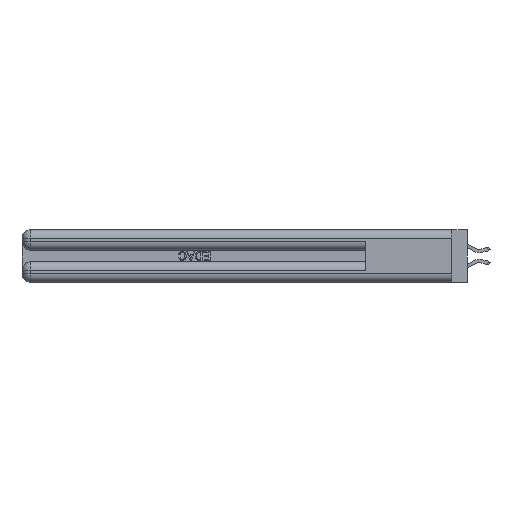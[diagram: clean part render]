
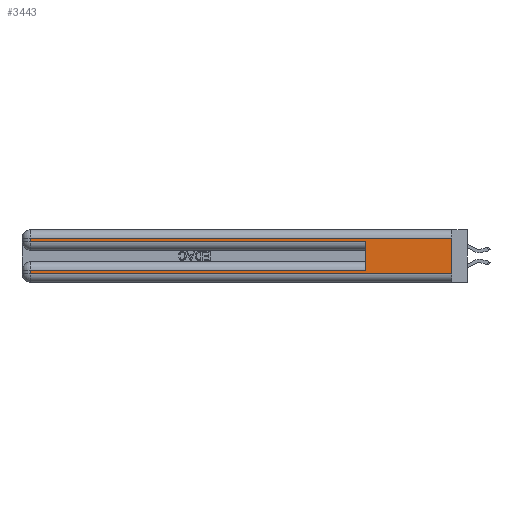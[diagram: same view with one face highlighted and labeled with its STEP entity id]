
A CAD part, left-side view. The second image highlights one B-rep face of the part: STEP entity #3443.
In plain terms, the highlighted planar face has unit normal (-1, 0, 0).
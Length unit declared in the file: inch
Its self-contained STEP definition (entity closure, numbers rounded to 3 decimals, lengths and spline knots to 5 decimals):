
#501 = EDGE_CURVE ( 'NONE', #843, #32070, #34687, .T. ) ;
#601 = CARTESIAN_POINT ( 'NONE',  ( 0., 2.94, 0.37 ) ) ;
#843 = VERTEX_POINT ( 'NONE', #7015 ) ;
#874 = DIRECTION ( 'NONE',  ( 1., 0., 0. ) ) ;
#916 = VECTOR ( 'NONE', #10515, 39.37008 ) ;
#2518 = LINE ( 'NONE', #15724, #18730 ) ;
#2704 = VECTOR ( 'NONE', #35633, 39.37008 ) ;
#3443 = ADVANCED_FACE ( 'NONE', ( #39910 ), #13935, .F. ) ;
#3871 = DIRECTION ( 'NONE',  ( 0., 0., -1. ) ) ;
#3936 = CARTESIAN_POINT ( 'NONE',  ( 0., 0., 0.085 ) ) ;
#3945 = EDGE_CURVE ( 'NONE', #12988, #25513, #35281, .T. ) ;
#5724 = VECTOR ( 'NONE', #37586, 39.37008 ) ;
#6409 = CARTESIAN_POINT ( 'NONE',  ( 0., 2.94, 0.06 ) ) ;
#6860 = EDGE_LOOP ( 'NONE', ( #8794, #41112, #40814, #14223, #36504, #16221, #21613, #37653 ) ) ;
#7015 = CARTESIAN_POINT ( 'NONE',  ( 0., 0.6, 0.085 ) ) ;
#8485 = EDGE_CURVE ( 'NONE', #843, #13185, #40941, .T. ) ;
#8794 = ORIENTED_EDGE ( 'NONE', *, *, #3945, .F. ) ;
#9988 = VECTOR ( 'NONE', #15255, 39.37008 ) ;
#10515 = DIRECTION ( 'NONE',  ( 0., 0., -1. ) ) ;
#10680 = CARTESIAN_POINT ( 'NONE',  ( 0., 0., 0.37 ) ) ;
#11206 = DIRECTION ( 'NONE',  ( 0., -1., 0. ) ) ;
#12092 = EDGE_CURVE ( 'NONE', #13185, #39303, #19924, .T. ) ;
#12988 = VERTEX_POINT ( 'NONE', #27149 ) ;
#13185 = VERTEX_POINT ( 'NONE', #18389 ) ;
#13935 = PLANE ( 'NONE',  #37952 ) ;
#14223 = ORIENTED_EDGE ( 'NONE', *, *, #25972, .T. ) ;
#14345 = LINE ( 'NONE', #34382, #5724 ) ;
#15255 = DIRECTION ( 'NONE',  ( 0., 0., 1. ) ) ;
#15724 = CARTESIAN_POINT ( 'NONE',  ( 0., 0., 0.285 ) ) ;
#16221 = ORIENTED_EDGE ( 'NONE', *, *, #8485, .T. ) ;
#16312 = CARTESIAN_POINT ( 'NONE',  ( 0., 2.94, 0.37 ) ) ;
#17136 = DIRECTION ( 'NONE',  ( 0., 0., -1. ) ) ;
#17548 = VECTOR ( 'NONE', #11206, 39.37008 ) ;
#18389 = CARTESIAN_POINT ( 'NONE',  ( 0., 2.94, 0.085 ) ) ;
#18730 = VECTOR ( 'NONE', #41468, 39.37008 ) ;
#19924 = LINE ( 'NONE', #16312, #2704 ) ;
#20411 = CARTESIAN_POINT ( 'NONE',  ( 0., 0.6, 0.285 ) ) ;
#21127 = LINE ( 'NONE', #601, #37200 ) ;
#21613 = ORIENTED_EDGE ( 'NONE', *, *, #12092, .T. ) ;
#22841 = VECTOR ( 'NONE', #26558, 39.37008 ) ;
#23289 = EDGE_CURVE ( 'NONE', #12988, #25600, #14345, .T. ) ;
#23323 = CARTESIAN_POINT ( 'NONE',  ( 0., 0., 0.37 ) ) ;
#25513 = VERTEX_POINT ( 'NONE', #25909 ) ;
#25600 = VERTEX_POINT ( 'NONE', #36453 ) ;
#25909 = CARTESIAN_POINT ( 'NONE',  ( 0., 0., 0.06 ) ) ;
#25972 = EDGE_CURVE ( 'NONE', #33109, #32070, #2518, .T. ) ;
#26558 = DIRECTION ( 'NONE',  ( 0., 1., 0. ) ) ;
#27149 = CARTESIAN_POINT ( 'NONE',  ( 0., 0., 0.31 ) ) ;
#27277 = CARTESIAN_POINT ( 'NONE',  ( 0., 0., 0.06 ) ) ;
#27539 = EDGE_CURVE ( 'NONE', #25600, #33109, #21127, .T. ) ;
#32070 = VERTEX_POINT ( 'NONE', #20411 ) ;
#33109 = VERTEX_POINT ( 'NONE', #41403 ) ;
#33687 = LINE ( 'NONE', #27277, #17548 ) ;
#34382 = CARTESIAN_POINT ( 'NONE',  ( 0., 0., 0.31 ) ) ;
#34569 = CARTESIAN_POINT ( 'NONE',  ( 0., 0.6, 0.145 ) ) ;
#34687 = LINE ( 'NONE', #34569, #9988 ) ;
#35281 = LINE ( 'NONE', #23323, #916 ) ;
#35633 = DIRECTION ( 'NONE',  ( 0., 0., -1. ) ) ;
#36453 = CARTESIAN_POINT ( 'NONE',  ( 0., 2.94, 0.31 ) ) ;
#36504 = ORIENTED_EDGE ( 'NONE', *, *, #501, .F. ) ;
#37200 = VECTOR ( 'NONE', #3871, 39.37008 ) ;
#37586 = DIRECTION ( 'NONE',  ( 0., 1., 0. ) ) ;
#37653 = ORIENTED_EDGE ( 'NONE', *, *, #40154, .T. ) ;
#37952 = AXIS2_PLACEMENT_3D ( 'NONE', #10680, #874, #17136 ) ;
#39303 = VERTEX_POINT ( 'NONE', #6409 ) ;
#39910 = FACE_OUTER_BOUND ( 'NONE', #6860, .T. ) ;
#40154 = EDGE_CURVE ( 'NONE', #39303, #25513, #33687, .T. ) ;
#40814 = ORIENTED_EDGE ( 'NONE', *, *, #27539, .T. ) ;
#40941 = LINE ( 'NONE', #3936, #22841 ) ;
#41112 = ORIENTED_EDGE ( 'NONE', *, *, #23289, .T. ) ;
#41403 = CARTESIAN_POINT ( 'NONE',  ( 0., 2.94, 0.285 ) ) ;
#41468 = DIRECTION ( 'NONE',  ( 0., -1., 0. ) ) ;
